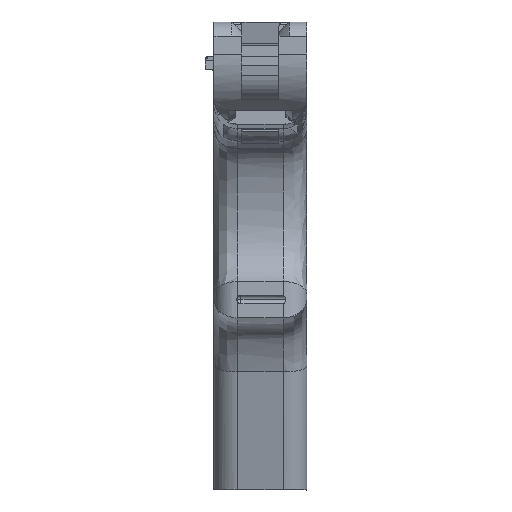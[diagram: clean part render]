
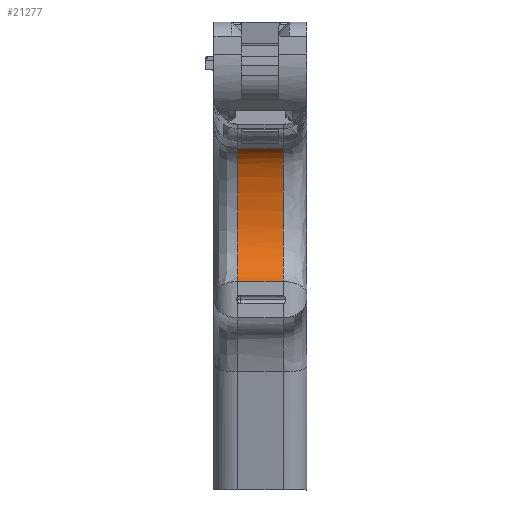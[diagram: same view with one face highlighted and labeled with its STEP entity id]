
A CAD part, front view. The second image highlights one B-rep face of the part: STEP entity #21277.
In plain terms, the highlighted free-form (B-spline) face has degree [5, 1] with [20, 2] control points.
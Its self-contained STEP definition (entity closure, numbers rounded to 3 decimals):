
#663=(
BOUNDED_SURFACE()
B_SPLINE_SURFACE(5,1,((#43869,#43870),(#43871,#43872),(#43873,#43874),(#43875,
#43876),(#43877,#43878),(#43879,#43880),(#43881,#43882),(#43883,#43884),
(#43885,#43886),(#43887,#43888),(#43889,#43890),(#43891,#43892),(#43893,
#43894),(#43895,#43896),(#43897,#43898),(#43899,#43900),(#43901,#43902),
(#43903,#43904),(#43905,#43906),(#43907,#43908)),.UNSPECIFIED.,.F.,.F.,
 .F.)
B_SPLINE_SURFACE_WITH_KNOTS((6,1,1,1,1,1,1,1,1,1,1,1,1,1,1,6),(2,2),(-1.,
-0.96,-0.92,-0.88,-0.84,-0.8,-0.76,-0.72,-0.68,-0.64,-0.6,-0.56,-0.52,-0.48,
-0.44,-0.423),(-6.5,6.5),.UNSPECIFIED.)
GEOMETRIC_REPRESENTATION_ITEM()
RATIONAL_B_SPLINE_SURFACE(((1.,1.),(1.,1.),(1.,1.),(1.,1.),(1.,1.),(1.,
1.),(1.,1.),(1.,1.),(1.,1.),(1.,1.),(1.,1.),(1.,1.),(1.,1.),(1.,1.),(1.,
1.),(1.,1.),(1.,1.),(1.,1.),(1.,1.),(1.,1.)))
REPRESENTATION_ITEM('')
SURFACE()
);
#2457=B_SPLINE_CURVE_WITH_KNOTS('',3,(#43663,#43664,#43665,#43666,#43667,
#43668,#43669,#43670,#43671,#43672,#43673,#43674),.UNSPECIFIED.,.F.,.F.,
(4,1,1,1,1,1,1,1,1,4),(0.,0.484,0.968,
1.452,1.936,2.177,2.419,2.903,
3.145,3.387),.UNSPECIFIED.);
#2461=B_SPLINE_CURVE_WITH_KNOTS('',3,(#43911,#43912,#43913,#43914,#43915,
#43916,#43917,#43918,#43919,#43920,#43921,#43922),.UNSPECIFIED.,.F.,.F.,
(4,1,1,1,1,1,1,1,1,4),(0.,0.242,0.363,0.484,
0.968,1.452,1.936,2.419,2.903,
3.387),.UNSPECIFIED.);
#3761=FACE_OUTER_BOUND('',#4979,.T.);
#4979=EDGE_LOOP('',(#19447,#19448,#19449,#19450));
#6300=LINE('',#43370,#7628);
#6343=LINE('',#43910,#7671);
#7628=VECTOR('',#24449,10.);
#7671=VECTOR('',#24584,10.);
#8615=VERTEX_POINT('',#27736);
#10129=VERTEX_POINT('',#42646);
#10208=VERTEX_POINT('',#43648);
#10211=VERTEX_POINT('',#43909);
#13320=EDGE_CURVE('',#8615,#10129,#6300,.T.);
#13379=EDGE_CURVE('',#10208,#8615,#2457,.T.);
#13386=EDGE_CURVE('',#10208,#10211,#6343,.T.);
#13387=EDGE_CURVE('',#10129,#10211,#2461,.T.);
#19447=ORIENTED_EDGE('',*,*,#13379,.F.);
#19448=ORIENTED_EDGE('',*,*,#13386,.T.);
#19449=ORIENTED_EDGE('',*,*,#13387,.F.);
#19450=ORIENTED_EDGE('',*,*,#13320,.F.);
#21277=ADVANCED_FACE('',(#3761),#663,.F.);
#24449=DIRECTION('',(1.,0.,0.));
#24584=DIRECTION('',(1.,0.,0.));
#27736=CARTESIAN_POINT('',(-3.991,-33.833,59.383));
#42646=CARTESIAN_POINT('',(3.709,-33.833,59.383));
#43370=CARTESIAN_POINT('',(0.,-33.833,59.383));
#43648=CARTESIAN_POINT('',(-3.991,-33.833,37.));
#43663=CARTESIAN_POINT('Ctrl Pts',(-3.991,-33.833,
37.));
#43664=CARTESIAN_POINT('Ctrl Pts',(-3.991,-32.807,
37.559));
#43665=CARTESIAN_POINT('Ctrl Pts',(-3.991,-31.061,
38.956));
#43666=CARTESIAN_POINT('Ctrl Pts',(-3.991,-29.426,
41.874));
#43667=CARTESIAN_POINT('Ctrl Pts',(-3.991,-28.795,
45.545));
#43668=CARTESIAN_POINT('Ctrl Pts',(-3.991,-29.034,
48.964));
#43669=CARTESIAN_POINT('Ctrl Pts',(-3.991,-29.568,
51.742));
#43670=CARTESIAN_POINT('Ctrl Pts',(-3.991,-30.306,
54.481));
#43671=CARTESIAN_POINT('Ctrl Pts',(-3.991,-31.322,
56.884));
#43672=CARTESIAN_POINT('Ctrl Pts',(-3.991,-32.6,
58.471));
#43673=CARTESIAN_POINT('Ctrl Pts',(-3.991,-33.385,
59.1));
#43674=CARTESIAN_POINT('Ctrl Pts',(-3.991,-33.833,
59.383));
#43869=CARTESIAN_POINT('Ctrl Pts',(-65.,-33.833,37.));
#43870=CARTESIAN_POINT('Ctrl Pts',(65.,-33.833,37.));
#43871=CARTESIAN_POINT('Ctrl Pts',(-65.,-33.535,37.162));
#43872=CARTESIAN_POINT('Ctrl Pts',(65.,-33.535,37.162));
#43873=CARTESIAN_POINT('Ctrl Pts',(-65.,-32.961,37.506));
#43874=CARTESIAN_POINT('Ctrl Pts',(65.,-32.961,37.506));
#43875=CARTESIAN_POINT('Ctrl Pts',(-65.,-32.168,38.078));
#43876=CARTESIAN_POINT('Ctrl Pts',(65.,-32.168,38.078));
#43877=CARTESIAN_POINT('Ctrl Pts',(-65.,-31.245,38.956));
#43878=CARTESIAN_POINT('Ctrl Pts',(65.,-31.245,38.956));
#43879=CARTESIAN_POINT('Ctrl Pts',(-65.,-30.319,40.243));
#43880=CARTESIAN_POINT('Ctrl Pts',(65.,-30.319,40.243));
#43881=CARTESIAN_POINT('Ctrl Pts',(-65.,-29.621,41.718));
#43882=CARTESIAN_POINT('Ctrl Pts',(65.,-29.621,41.718));
#43883=CARTESIAN_POINT('Ctrl Pts',(-65.,-29.153,43.372));
#43884=CARTESIAN_POINT('Ctrl Pts',(65.,-29.153,43.372));
#43885=CARTESIAN_POINT('Ctrl Pts',(-65.,-28.915,45.19));
#43886=CARTESIAN_POINT('Ctrl Pts',(65.,-28.915,45.19));
#43887=CARTESIAN_POINT('Ctrl Pts',(-65.,-28.897,47.141));
#43888=CARTESIAN_POINT('Ctrl Pts',(65.,-28.897,47.141));
#43889=CARTESIAN_POINT('Ctrl Pts',(-65.,-29.084,49.178));
#43890=CARTESIAN_POINT('Ctrl Pts',(65.,-29.084,49.178));
#43891=CARTESIAN_POINT('Ctrl Pts',(-65.,-29.444,51.23));
#43892=CARTESIAN_POINT('Ctrl Pts',(65.,-29.444,51.23));
#43893=CARTESIAN_POINT('Ctrl Pts',(-65.,-29.937,53.208));
#43894=CARTESIAN_POINT('Ctrl Pts',(65.,-29.937,53.208));
#43895=CARTESIAN_POINT('Ctrl Pts',(-65.,-30.537,55.026));
#43896=CARTESIAN_POINT('Ctrl Pts',(65.,-30.537,55.026));
#43897=CARTESIAN_POINT('Ctrl Pts',(-65.,-31.24,56.616));
#43898=CARTESIAN_POINT('Ctrl Pts',(65.,-31.24,56.616));
#43899=CARTESIAN_POINT('Ctrl Pts',(-65.,-31.991,57.795));
#43900=CARTESIAN_POINT('Ctrl Pts',(65.,-31.991,57.795));
#43901=CARTESIAN_POINT('Ctrl Pts',(-65.,-32.711,58.563));
#43902=CARTESIAN_POINT('Ctrl Pts',(65.,-32.711,58.563));
#43903=CARTESIAN_POINT('Ctrl Pts',(-65.,-33.317,59.044));
#43904=CARTESIAN_POINT('Ctrl Pts',(65.,-33.317,59.044));
#43905=CARTESIAN_POINT('Ctrl Pts',(-65.,-33.712,59.306));
#43906=CARTESIAN_POINT('Ctrl Pts',(65.,-33.712,59.306));
#43907=CARTESIAN_POINT('Ctrl Pts',(-65.,-33.833,59.383));
#43908=CARTESIAN_POINT('Ctrl Pts',(65.,-33.833,59.383));
#43909=CARTESIAN_POINT('',(3.709,-33.833,37.));
#43910=CARTESIAN_POINT('',(0.,-33.833,37.));
#43911=CARTESIAN_POINT('Ctrl Pts',(3.709,-33.833,59.383));
#43912=CARTESIAN_POINT('Ctrl Pts',(3.709,-33.385,59.1));
#43913=CARTESIAN_POINT('Ctrl Pts',(3.709,-32.796,58.634));
#43914=CARTESIAN_POINT('Ctrl Pts',(3.709,-32.121,57.876));
#43915=CARTESIAN_POINT('Ctrl Pts',(3.709,-31.195,56.591));
#43916=CARTESIAN_POINT('Ctrl Pts',(3.709,-30.052,53.861));
#43917=CARTESIAN_POINT('Ctrl Pts',(3.709,-29.082,49.633));
#43918=CARTESIAN_POINT('Ctrl Pts',(3.709,-28.794,45.549));
#43919=CARTESIAN_POINT('Ctrl Pts',(3.709,-29.426,41.87));
#43920=CARTESIAN_POINT('Ctrl Pts',(3.709,-31.061,38.956));
#43921=CARTESIAN_POINT('Ctrl Pts',(3.709,-32.807,37.559));
#43922=CARTESIAN_POINT('Ctrl Pts',(3.709,-33.833,37.));
